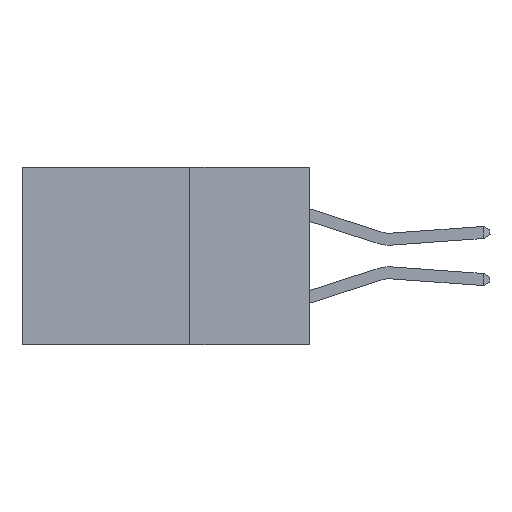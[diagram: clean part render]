
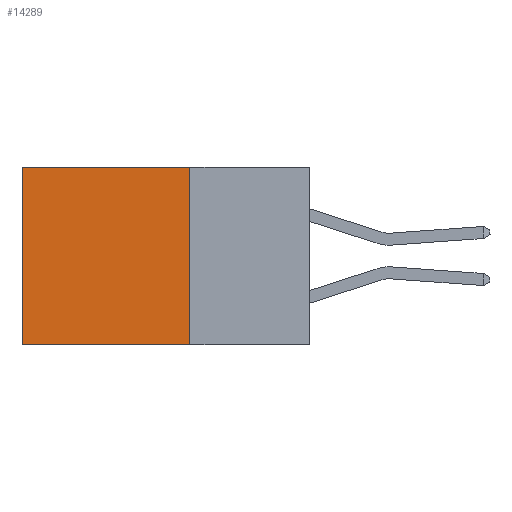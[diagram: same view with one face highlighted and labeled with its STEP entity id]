
A CAD part, left-side view. The second image highlights one B-rep face of the part: STEP entity #14289.
In plain terms, the highlighted planar face has unit normal (-1, 0, 0).
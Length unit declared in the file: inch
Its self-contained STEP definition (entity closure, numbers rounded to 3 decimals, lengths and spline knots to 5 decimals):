
#2883 = CARTESIAN_POINT ( 'NONE',  ( 0.298, 0.25, 0. ) ) ;
#2908 = DIRECTION ( 'NONE',  ( 0., 0., -1. ) ) ;
#3851 = VERTEX_POINT ( 'NONE', #22582 ) ;
#5329 = EDGE_CURVE ( 'NONE', #24013, #14927, #15277, .T. ) ;
#5669 = VERTEX_POINT ( 'NONE', #12180 ) ;
#6250 = LINE ( 'NONE', #24447, #19055 ) ;
#6598 = FACE_OUTER_BOUND ( 'NONE', #8358, .T. ) ;
#7496 = DIRECTION ( 'NONE',  ( 1., 0., 0. ) ) ;
#7698 = EDGE_CURVE ( 'NONE', #24013, #3851, #20277, .T. ) ;
#8358 = EDGE_LOOP ( 'NONE', ( #16088, #26973, #27863, #29163 ) ) ;
#12180 = CARTESIAN_POINT ( 'NONE',  ( 0.298, 0.6, -0.37 ) ) ;
#12481 = VECTOR ( 'NONE', #15200, 39.37008 ) ;
#13241 = DIRECTION ( 'NONE',  ( 0., 1., 0. ) ) ;
#14289 = ADVANCED_FACE ( 'NONE', ( #6598 ), #16579, .F. ) ;
#14310 = CARTESIAN_POINT ( 'NONE',  ( 0.298, 0.25, 0. ) ) ;
#14554 = VECTOR ( 'NONE', #24881, 39.37008 ) ;
#14668 = LINE ( 'NONE', #21871, #12481 ) ;
#14927 = VERTEX_POINT ( 'NONE', #27392 ) ;
#15200 = DIRECTION ( 'NONE',  ( 0., 0., -1. ) ) ;
#15277 = LINE ( 'NONE', #24490, #14554 ) ;
#16088 = ORIENTED_EDGE ( 'NONE', *, *, #20482, .T. ) ;
#16372 = CARTESIAN_POINT ( 'NONE',  ( 0.298, 0.25, 0. ) ) ;
#16579 = PLANE ( 'NONE',  #28338 ) ;
#19055 = VECTOR ( 'NONE', #13241, 39.37008 ) ;
#19597 = VECTOR ( 'NONE', #2908, 39.37008 ) ;
#20277 = LINE ( 'NONE', #14310, #19597 ) ;
#20482 = EDGE_CURVE ( 'NONE', #14927, #5669, #14668, .T. ) ;
#21871 = CARTESIAN_POINT ( 'NONE',  ( 0.298, 0.6, 0. ) ) ;
#22582 = CARTESIAN_POINT ( 'NONE',  ( 0.298, 0.25, -0.37 ) ) ;
#23308 = DIRECTION ( 'NONE',  ( 0., 0., -1. ) ) ;
#24013 = VERTEX_POINT ( 'NONE', #16372 ) ;
#24435 = EDGE_CURVE ( 'NONE', #3851, #5669, #6250, .T. ) ;
#24447 = CARTESIAN_POINT ( 'NONE',  ( 0.298, 0.25, -0.37 ) ) ;
#24490 = CARTESIAN_POINT ( 'NONE',  ( 0.298, 0.25, 0. ) ) ;
#24881 = DIRECTION ( 'NONE',  ( 0., 1., 0. ) ) ;
#26973 = ORIENTED_EDGE ( 'NONE', *, *, #24435, .F. ) ;
#27392 = CARTESIAN_POINT ( 'NONE',  ( 0.298, 0.6, 0. ) ) ;
#27863 = ORIENTED_EDGE ( 'NONE', *, *, #7698, .F. ) ;
#28338 = AXIS2_PLACEMENT_3D ( 'NONE', #2883, #7496, #23308 ) ;
#29163 = ORIENTED_EDGE ( 'NONE', *, *, #5329, .T. ) ;
